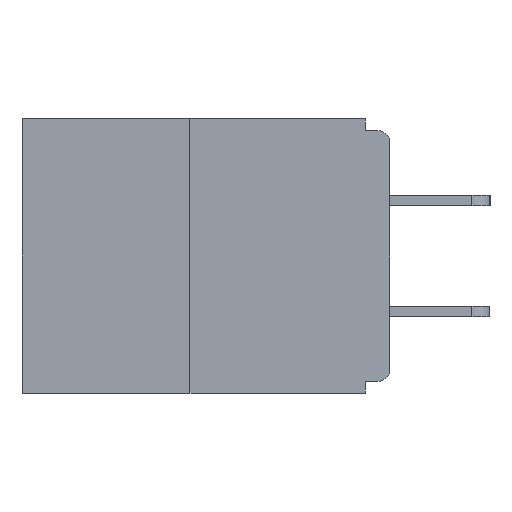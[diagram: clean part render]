
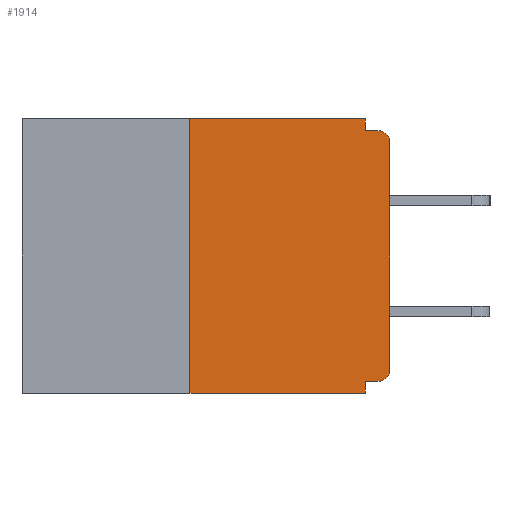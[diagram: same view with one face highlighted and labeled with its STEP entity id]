
A CAD part, left-side view. The second image highlights one B-rep face of the part: STEP entity #1914.
In plain terms, the highlighted planar face has unit normal (-1, 0, 0).
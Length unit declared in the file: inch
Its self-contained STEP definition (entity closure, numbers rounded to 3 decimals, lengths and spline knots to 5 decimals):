
#80 = EDGE_CURVE ( 'NONE', #12187, #7020, #9026, .T. ) ;
#144 = CARTESIAN_POINT ( 'NONE',  ( 0., 0.015, -0.03 ) ) ;
#172 = ORIENTED_EDGE ( 'NONE', *, *, #2592, .F. ) ;
#375 = DIRECTION ( 'NONE',  ( 0., 0., 1. ) ) ;
#670 = LINE ( 'NONE', #7512, #13533 ) ;
#1042 = CARTESIAN_POINT ( 'NONE',  ( 0., 0.46, 0. ) ) ;
#1055 = EDGE_CURVE ( 'NONE', #3249, #9279, #10082, .T. ) ;
#1108 = ORIENTED_EDGE ( 'NONE', *, *, #14649, .T. ) ;
#1314 = ORIENTED_EDGE ( 'NONE', *, *, #10935, .F. ) ;
#1359 = VERTEX_POINT ( 'NONE', #13416 ) ;
#1448 = ORIENTED_EDGE ( 'NONE', *, *, #6962, .F. ) ;
#1581 = DIRECTION ( 'NONE',  ( -1., 0., 0. ) ) ;
#1776 = DIRECTION ( 'NONE',  ( 0., 1., 0. ) ) ;
#1907 = AXIS2_PLACEMENT_3D ( 'NONE', #12408, #14776, #3192 ) ;
#1908 = VERTEX_POINT ( 'NONE', #7699 ) ;
#1914 = ADVANCED_FACE ( 'NONE', ( #3119 ), #7769, .F. ) ;
#1915 = CARTESIAN_POINT ( 'NONE',  ( 0., 0.46, -0.343 ) ) ;
#2005 = VECTOR ( 'NONE', #375, 39.37008 ) ;
#2592 = EDGE_CURVE ( 'NONE', #4647, #1908, #7676, .T. ) ;
#2852 = EDGE_CURVE ( 'NONE', #4930, #3249, #11468, .T. ) ;
#2965 = LINE ( 'NONE', #1915, #3498 ) ;
#3119 = FACE_OUTER_BOUND ( 'NONE', #11765, .T. ) ;
#3192 = DIRECTION ( 'NONE',  ( 0., 0., -1. ) ) ;
#3249 = VERTEX_POINT ( 'NONE', #11503 ) ;
#3319 = CARTESIAN_POINT ( 'NONE',  ( 0., 0., 0. ) ) ;
#3375 = VERTEX_POINT ( 'NONE', #12109 ) ;
#3395 = CARTESIAN_POINT ( 'NONE',  ( 0., 0.031, -0.328 ) ) ;
#3498 = VECTOR ( 'NONE', #7618, 39.37008 ) ;
#3600 = VECTOR ( 'NONE', #14752, 39.37008 ) ;
#3629 = DIRECTION ( 'NONE',  ( 0., 0., -1. ) ) ;
#3658 = CARTESIAN_POINT ( 'NONE',  ( 0., 0.015, -0.328 ) ) ;
#3759 = ORIENTED_EDGE ( 'NONE', *, *, #80, .T. ) ;
#4026 = CARTESIAN_POINT ( 'NONE',  ( 0., 0.031, -0.343 ) ) ;
#4157 = VERTEX_POINT ( 'NONE', #7339 ) ;
#4340 = VECTOR ( 'NONE', #12757, 39.37008 ) ;
#4441 = CARTESIAN_POINT ( 'NONE',  ( 0., 0.25, 0. ) ) ;
#4647 = VERTEX_POINT ( 'NONE', #3395 ) ;
#4930 = VERTEX_POINT ( 'NONE', #4441 ) ;
#5237 = DIRECTION ( 'NONE',  ( -1., 0., 0. ) ) ;
#5359 = EDGE_CURVE ( 'NONE', #12187, #4647, #14634, .T. ) ;
#6394 = AXIS2_PLACEMENT_3D ( 'NONE', #144, #1581, #3629 ) ;
#6536 = VECTOR ( 'NONE', #10229, 39.37008 ) ;
#6739 = CARTESIAN_POINT ( 'NONE',  ( 0., 0., -0.313 ) ) ;
#6962 = EDGE_CURVE ( 'NONE', #9279, #1359, #670, .T. ) ;
#7020 = VERTEX_POINT ( 'NONE', #6739 ) ;
#7339 = CARTESIAN_POINT ( 'NONE',  ( 0., 0.25, -0.343 ) ) ;
#7444 = LINE ( 'NONE', #9647, #2005 ) ;
#7512 = CARTESIAN_POINT ( 'NONE',  ( 0., 0., -0.015 ) ) ;
#7618 = DIRECTION ( 'NONE',  ( 0., -1., 0. ) ) ;
#7676 = LINE ( 'NONE', #4026, #3600 ) ;
#7699 = CARTESIAN_POINT ( 'NONE',  ( 0., 0.031, -0.343 ) ) ;
#7769 = PLANE ( 'NONE',  #1907 ) ;
#8738 = DIRECTION ( 'NONE',  ( 0., -1., 0. ) ) ;
#8771 = CARTESIAN_POINT ( 'NONE',  ( 0., 0., -0.328 ) ) ;
#9026 = CIRCLE ( 'NONE', #13111, 0.015 ) ;
#9174 = CARTESIAN_POINT ( 'NONE',  ( 0., 0.031, 0. ) ) ;
#9279 = VERTEX_POINT ( 'NONE', #14230 ) ;
#9647 = CARTESIAN_POINT ( 'NONE',  ( 0., 0.25, 0. ) ) ;
#9717 = ORIENTED_EDGE ( 'NONE', *, *, #5359, .F. ) ;
#9875 = CARTESIAN_POINT ( 'NONE',  ( 0., 0.015, -0.313 ) ) ;
#10034 = ORIENTED_EDGE ( 'NONE', *, *, #11673, .T. ) ;
#10082 = LINE ( 'NONE', #9174, #6536 ) ;
#10229 = DIRECTION ( 'NONE',  ( 0., 0., -1. ) ) ;
#10935 = EDGE_CURVE ( 'NONE', #4157, #4930, #7444, .T. ) ;
#11079 = VECTOR ( 'NONE', #1776, 39.37008 ) ;
#11296 = ORIENTED_EDGE ( 'NONE', *, *, #13045, .T. ) ;
#11468 = LINE ( 'NONE', #1042, #4340 ) ;
#11503 = CARTESIAN_POINT ( 'NONE',  ( 0., 0.031, 0. ) ) ;
#11673 = EDGE_CURVE ( 'NONE', #7020, #3375, #14036, .T. ) ;
#11746 = DIRECTION ( 'NONE',  ( 0., 0., 1. ) ) ;
#11765 = EDGE_LOOP ( 'NONE', ( #13819, #1314, #11296, #172, #9717, #3759, #10034, #1108, #1448, #14877 ) ) ;
#12109 = CARTESIAN_POINT ( 'NONE',  ( 0., 0., -0.03 ) ) ;
#12187 = VERTEX_POINT ( 'NONE', #3658 ) ;
#12408 = CARTESIAN_POINT ( 'NONE',  ( 0., 0.46, 0. ) ) ;
#12757 = DIRECTION ( 'NONE',  ( 0., -1., 0. ) ) ;
#12957 = VECTOR ( 'NONE', #11746, 39.37008 ) ;
#13045 = EDGE_CURVE ( 'NONE', #4157, #1908, #2965, .T. ) ;
#13111 = AXIS2_PLACEMENT_3D ( 'NONE', #9875, #5237, #14535 ) ;
#13416 = CARTESIAN_POINT ( 'NONE',  ( 0., 0.015, -0.015 ) ) ;
#13533 = VECTOR ( 'NONE', #8738, 39.37008 ) ;
#13819 = ORIENTED_EDGE ( 'NONE', *, *, #2852, .F. ) ;
#13932 = CIRCLE ( 'NONE', #6394, 0.015 ) ;
#14036 = LINE ( 'NONE', #3319, #12957 ) ;
#14230 = CARTESIAN_POINT ( 'NONE',  ( 0., 0.031, -0.015 ) ) ;
#14535 = DIRECTION ( 'NONE',  ( 0., 0., -1. ) ) ;
#14634 = LINE ( 'NONE', #8771, #11079 ) ;
#14649 = EDGE_CURVE ( 'NONE', #3375, #1359, #13932, .T. ) ;
#14752 = DIRECTION ( 'NONE',  ( 0., 0., -1. ) ) ;
#14776 = DIRECTION ( 'NONE',  ( 1., 0., 0. ) ) ;
#14877 = ORIENTED_EDGE ( 'NONE', *, *, #1055, .F. ) ;
